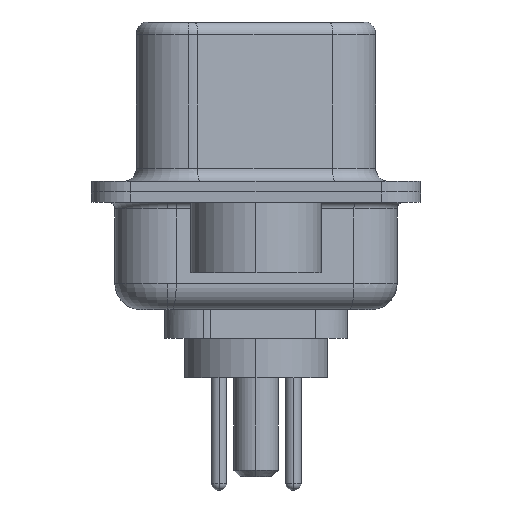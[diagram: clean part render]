
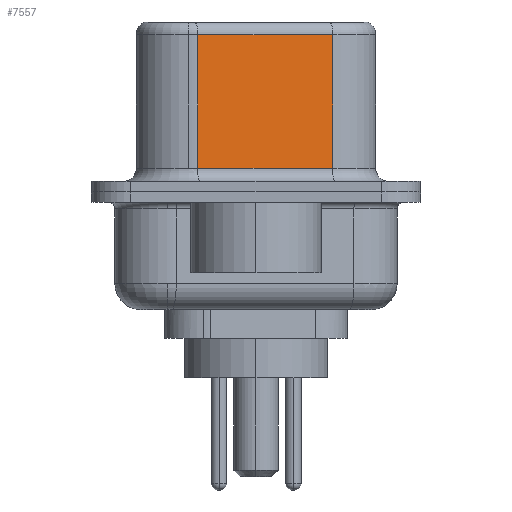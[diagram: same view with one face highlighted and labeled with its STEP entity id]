
A CAD part, left-side view. The second image highlights one B-rep face of the part: STEP entity #7557.
In plain terms, the highlighted planar face has unit normal (-0.985, -0.174, 0).
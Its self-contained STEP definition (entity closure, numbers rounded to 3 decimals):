
#230 = CARTESIAN_POINT ( 'NONE',  ( 4.585, -2.927, 0.9 ) ) ;
#1136 = VERTEX_POINT ( 'NONE', #15440 ) ;
#1550 = ORIENTED_EDGE ( 'NONE', *, *, #14632, .T. ) ;
#2572 = DIRECTION ( 'NONE',  ( 0.985, 0.174, 0. ) ) ;
#3439 = DIRECTION ( 'NONE',  ( -0.174, 0.985, 0. ) ) ;
#4018 = VECTOR ( 'NONE', #3439, 1000. ) ;
#4048 = EDGE_CURVE ( 'NONE', #1136, #5141, #7521, .T. ) ;
#4209 = EDGE_LOOP ( 'NONE', ( #11807, #13609, #1550, #12738 ) ) ;
#5141 = VERTEX_POINT ( 'NONE', #230 ) ;
#5388 = AXIS2_PLACEMENT_3D ( 'NONE', #10511, #2572, #11869 ) ;
#5594 = VECTOR ( 'NONE', #17123, 1000. ) ;
#6018 = CARTESIAN_POINT ( 'NONE',  ( 4.585, -2.927, 6.02 ) ) ;
#6060 = VECTOR ( 'NONE', #11377, 1000. ) ;
#6090 = EDGE_CURVE ( 'NONE', #15663, #5141, #15778, .T. ) ;
#6094 = CARTESIAN_POINT ( 'NONE',  ( 4.585, -2.927, 6.02 ) ) ;
#6310 = FACE_OUTER_BOUND ( 'NONE', #4209, .T. ) ;
#6573 = VERTEX_POINT ( 'NONE', #7563 ) ;
#7521 = LINE ( 'NONE', #10973, #14193 ) ;
#7536 = LINE ( 'NONE', #6018, #4018 ) ;
#7557 = ADVANCED_FACE ( 'NONE', ( #6310 ), #7818, .F. ) ;
#7563 = CARTESIAN_POINT ( 'NONE',  ( 3.675, 2.233, 6.02 ) ) ;
#7818 = PLANE ( 'NONE',  #5388 ) ;
#7872 = CARTESIAN_POINT ( 'NONE',  ( 4.585, -2.927, 6.52 ) ) ;
#10011 = CARTESIAN_POINT ( 'NONE',  ( 3.675, 2.233, 6.52 ) ) ;
#10511 = CARTESIAN_POINT ( 'NONE',  ( 4.585, -2.927, 6.52 ) ) ;
#10973 = CARTESIAN_POINT ( 'NONE',  ( 4.585, -2.927, 0.9 ) ) ;
#11377 = DIRECTION ( 'NONE',  ( 0., 0., -1. ) ) ;
#11807 = ORIENTED_EDGE ( 'NONE', *, *, #6090, .F. ) ;
#11869 = DIRECTION ( 'NONE',  ( -0.174, 0.985, 0. ) ) ;
#12311 = DIRECTION ( 'NONE',  ( 0.174, -0.985, 0. ) ) ;
#12738 = ORIENTED_EDGE ( 'NONE', *, *, #4048, .T. ) ;
#13609 = ORIENTED_EDGE ( 'NONE', *, *, #14250, .T. ) ;
#14193 = VECTOR ( 'NONE', #12311, 1000. ) ;
#14250 = EDGE_CURVE ( 'NONE', #15663, #6573, #7536, .T. ) ;
#14632 = EDGE_CURVE ( 'NONE', #6573, #1136, #16632, .T. ) ;
#15440 = CARTESIAN_POINT ( 'NONE',  ( 3.675, 2.233, 0.9 ) ) ;
#15663 = VERTEX_POINT ( 'NONE', #6094 ) ;
#15778 = LINE ( 'NONE', #7872, #5594 ) ;
#16632 = LINE ( 'NONE', #10011, #6060 ) ;
#17123 = DIRECTION ( 'NONE',  ( 0., 0., -1. ) ) ;
